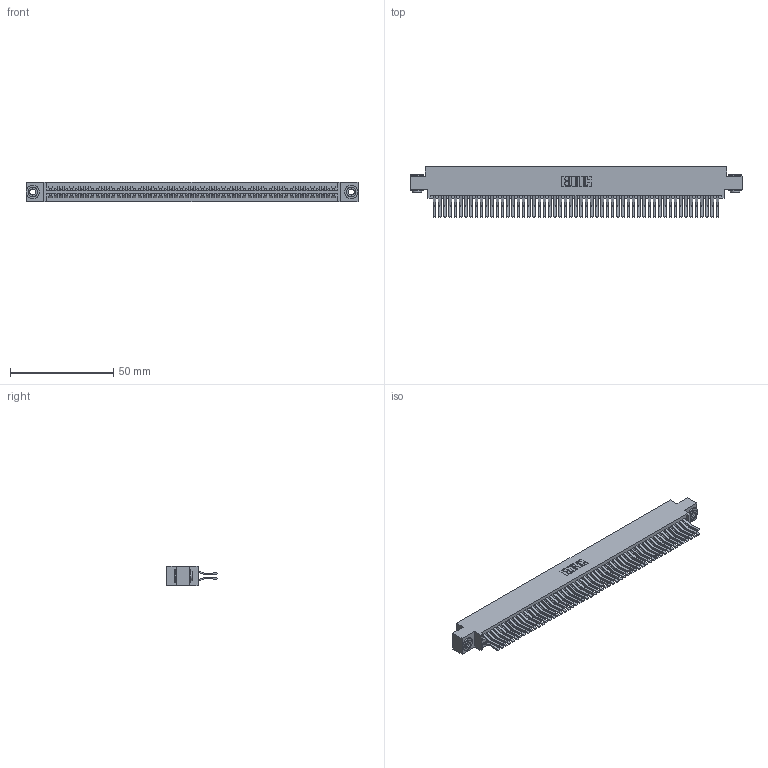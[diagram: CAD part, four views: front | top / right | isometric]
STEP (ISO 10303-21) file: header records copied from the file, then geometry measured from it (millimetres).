
FILE_DESCRIPTION (( 'STEP AP203' ), '1' );
FILE_NAME ('345-110-560-803.STEP', '2019-11-04T19:26:49', ( '' ), ( '' ), 'SwSTEP 2.0', 'SolidWorks 2016', '' );
FILE_SCHEMA (( 'CONFIG_CONTROL_DESIGN' ));
Length unit declared in the file: inch
Products named in the file (4): 345-292-001_560 Tail; 345 Part_0.170 Offset - 0.156 Dia-TH; 345-110-560-803; 345-250-002_345-250-002-102
Assembly tree (113 placements, depth 2):
  345-110-560-803
    345 Part_0.170 Offset - 0.156 Dia-TH
    345-292-001_560 Tail  x110
    345-250-002_345-250-002-102  x2
Bounding box: 160.91 x 24.45 x 9.4 mm (x, y, z)
Volume: 16378.6 mm3; surface area: 26664.8 mm2
Topology: 113 solids, 113 shells, 5888 faces, 17479 edges, 11502 vertices
Faces by surface type: plane 3724, cylinder 2156, cone 8
Entity records: 42274 total; most frequent: CARTESIAN_POINT 7051, ORIENTED_EDGE 6978, DIRECTION 6235, EDGE_CURVE 3489, VECTOR 3109, LINE 3109, VERTEX_POINT 2322, AXIS2_PLACEMENT_3D 1563
